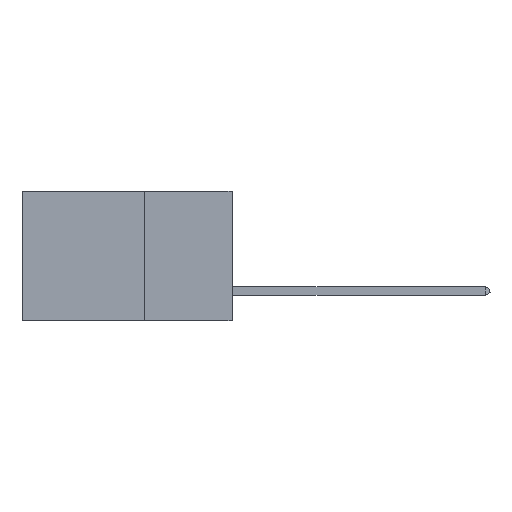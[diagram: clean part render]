
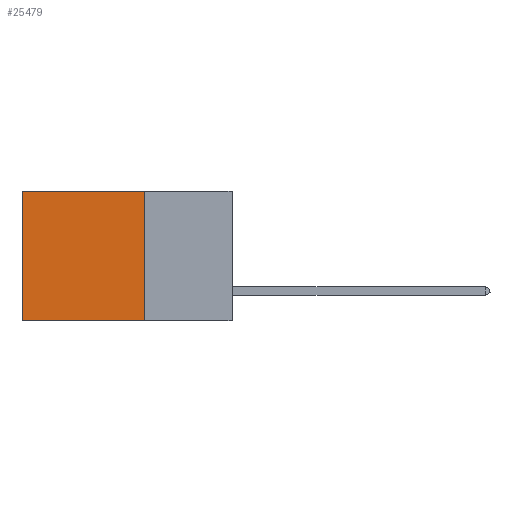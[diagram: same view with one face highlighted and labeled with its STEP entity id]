
A CAD part, left-side view. The second image highlights one B-rep face of the part: STEP entity #25479.
In plain terms, the highlighted planar face has unit normal (-1, 0, 0).
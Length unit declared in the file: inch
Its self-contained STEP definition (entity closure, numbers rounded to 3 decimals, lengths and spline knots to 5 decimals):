
#250 = CARTESIAN_POINT ( 'NONE',  ( 0.2875, 0.25, 0. ) ) ;
#524 = VERTEX_POINT ( 'NONE', #13601 ) ;
#573 = ORIENTED_EDGE ( 'NONE', *, *, #26223, .T. ) ;
#639 = EDGE_LOOP ( 'NONE', ( #1748, #15479, #13135, #573 ) ) ;
#1503 = LINE ( 'NONE', #250, #14382 ) ;
#1748 = ORIENTED_EDGE ( 'NONE', *, *, #12277, .T. ) ;
#4600 = LINE ( 'NONE', #28509, #15736 ) ;
#5039 = VERTEX_POINT ( 'NONE', #8417 ) ;
#6362 = VERTEX_POINT ( 'NONE', #27996 ) ;
#6510 = DIRECTION ( 'NONE',  ( 0., 0., -1. ) ) ;
#8417 = CARTESIAN_POINT ( 'NONE',  ( 0.2875, 0.6, 0. ) ) ;
#9020 = DIRECTION ( 'NONE',  ( 1., 0., 0. ) ) ;
#9411 = CARTESIAN_POINT ( 'NONE',  ( 0.2875, 0.25, -0.37 ) ) ;
#12277 = EDGE_CURVE ( 'NONE', #5039, #6362, #25119, .T. ) ;
#13135 = ORIENTED_EDGE ( 'NONE', *, *, #23357, .F. ) ;
#13515 = CARTESIAN_POINT ( 'NONE',  ( 0.2875, 0.25, 0. ) ) ;
#13601 = CARTESIAN_POINT ( 'NONE',  ( 0.2875, 0.25, 0. ) ) ;
#13795 = DIRECTION ( 'NONE',  ( 0., 1., 0. ) ) ;
#14382 = VECTOR ( 'NONE', #13795, 39.37008 ) ;
#14969 = VECTOR ( 'NONE', #6510, 39.37008 ) ;
#15479 = ORIENTED_EDGE ( 'NONE', *, *, #23038, .F. ) ;
#15736 = VECTOR ( 'NONE', #19349, 39.37008 ) ;
#16853 = DIRECTION ( 'NONE',  ( 0., 0., -1. ) ) ;
#17332 = FACE_OUTER_BOUND ( 'NONE', #639, .T. ) ;
#18100 = DIRECTION ( 'NONE',  ( 0., 0., -1. ) ) ;
#19349 = DIRECTION ( 'NONE',  ( 0., 1., 0. ) ) ;
#20922 = AXIS2_PLACEMENT_3D ( 'NONE', #27608, #9020, #18100 ) ;
#21051 = LINE ( 'NONE', #13515, #14969 ) ;
#22269 = VECTOR ( 'NONE', #16853, 39.37008 ) ;
#23038 = EDGE_CURVE ( 'NONE', #29542, #6362, #4600, .T. ) ;
#23357 = EDGE_CURVE ( 'NONE', #524, #29542, #21051, .T. ) ;
#25119 = LINE ( 'NONE', #25882, #22269 ) ;
#25283 = PLANE ( 'NONE',  #20922 ) ;
#25479 = ADVANCED_FACE ( 'NONE', ( #17332 ), #25283, .F. ) ;
#25882 = CARTESIAN_POINT ( 'NONE',  ( 0.2875, 0.6, 0. ) ) ;
#26223 = EDGE_CURVE ( 'NONE', #524, #5039, #1503, .T. ) ;
#27608 = CARTESIAN_POINT ( 'NONE',  ( 0.2875, 0.25, 0. ) ) ;
#27996 = CARTESIAN_POINT ( 'NONE',  ( 0.2875, 0.6, -0.37 ) ) ;
#28509 = CARTESIAN_POINT ( 'NONE',  ( 0.2875, 0.25, -0.37 ) ) ;
#29542 = VERTEX_POINT ( 'NONE', #9411 ) ;
